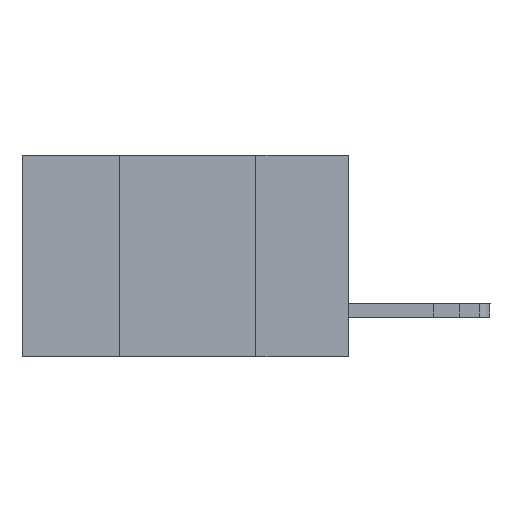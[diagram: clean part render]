
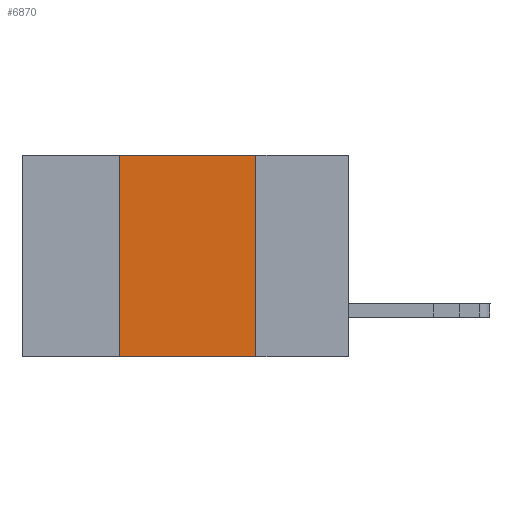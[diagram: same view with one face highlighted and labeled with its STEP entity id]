
A CAD part, left-side view. The second image highlights one B-rep face of the part: STEP entity #6870.
In plain terms, the highlighted planar face has unit normal (-1, 0, 0).
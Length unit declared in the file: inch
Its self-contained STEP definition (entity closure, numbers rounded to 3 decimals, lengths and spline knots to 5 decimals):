
#71 = AXIS2_PLACEMENT_3D ( 'NONE', #7877, #5910, #4125 ) ;
#196 = CARTESIAN_POINT ( 'NONE',  ( 0., 0.42, 0. ) ) ;
#542 = LINE ( 'NONE', #11119, #2959 ) ;
#704 = EDGE_CURVE ( 'NONE', #3866, #2626, #5231, .T. ) ;
#1407 = PLANE ( 'NONE',  #71 ) ;
#1589 = CARTESIAN_POINT ( 'NONE',  ( 0., 0.6, -0.37 ) ) ;
#2520 = DIRECTION ( 'NONE',  ( 0., 0., 1. ) ) ;
#2626 = VERTEX_POINT ( 'NONE', #10812 ) ;
#2959 = VECTOR ( 'NONE', #2520, 39.37008 ) ;
#2966 = VECTOR ( 'NONE', #8373, 39.37008 ) ;
#2983 = VERTEX_POINT ( 'NONE', #7077 ) ;
#3253 = EDGE_CURVE ( 'NONE', #3731, #2983, #4052, .T. ) ;
#3271 = ORIENTED_EDGE ( 'NONE', *, *, #8497, .F. ) ;
#3731 = VERTEX_POINT ( 'NONE', #196 ) ;
#3866 = VERTEX_POINT ( 'NONE', #9834 ) ;
#3986 = DIRECTION ( 'NONE',  ( 0., -1., 0. ) ) ;
#4052 = LINE ( 'NONE', #9610, #12030 ) ;
#4125 = DIRECTION ( 'NONE',  ( 0., 0., -1. ) ) ;
#4436 = DIRECTION ( 'NONE',  ( 0., -1., 0. ) ) ;
#4620 = LINE ( 'NONE', #11296, #2966 ) ;
#5231 = LINE ( 'NONE', #1589, #12033 ) ;
#5910 = DIRECTION ( 'NONE',  ( 1., 0., 0. ) ) ;
#6325 = ORIENTED_EDGE ( 'NONE', *, *, #8668, .F. ) ;
#6870 = ADVANCED_FACE ( 'NONE', ( #8871 ), #1407, .F. ) ;
#7077 = CARTESIAN_POINT ( 'NONE',  ( 0., 0.17, 0. ) ) ;
#7089 = ORIENTED_EDGE ( 'NONE', *, *, #704, .T. ) ;
#7451 = EDGE_LOOP ( 'NONE', ( #6325, #7454, #3271, #7089 ) ) ;
#7454 = ORIENTED_EDGE ( 'NONE', *, *, #3253, .F. ) ;
#7877 = CARTESIAN_POINT ( 'NONE',  ( 0., 0.6, 0. ) ) ;
#8373 = DIRECTION ( 'NONE',  ( 0., 0., -1. ) ) ;
#8497 = EDGE_CURVE ( 'NONE', #3866, #3731, #542, .T. ) ;
#8668 = EDGE_CURVE ( 'NONE', #2983, #2626, #4620, .T. ) ;
#8871 = FACE_OUTER_BOUND ( 'NONE', #7451, .T. ) ;
#9610 = CARTESIAN_POINT ( 'NONE',  ( 0., 0.6, 0. ) ) ;
#9834 = CARTESIAN_POINT ( 'NONE',  ( 0., 0.42, -0.37 ) ) ;
#10812 = CARTESIAN_POINT ( 'NONE',  ( 0., 0.17, -0.37 ) ) ;
#11119 = CARTESIAN_POINT ( 'NONE',  ( 0., 0.42, 0. ) ) ;
#11296 = CARTESIAN_POINT ( 'NONE',  ( 0., 0.17, 0. ) ) ;
#12030 = VECTOR ( 'NONE', #3986, 39.37008 ) ;
#12033 = VECTOR ( 'NONE', #4436, 39.37008 ) ;
